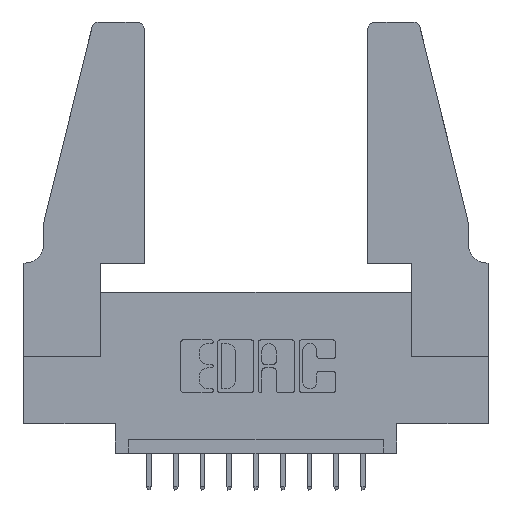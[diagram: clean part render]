
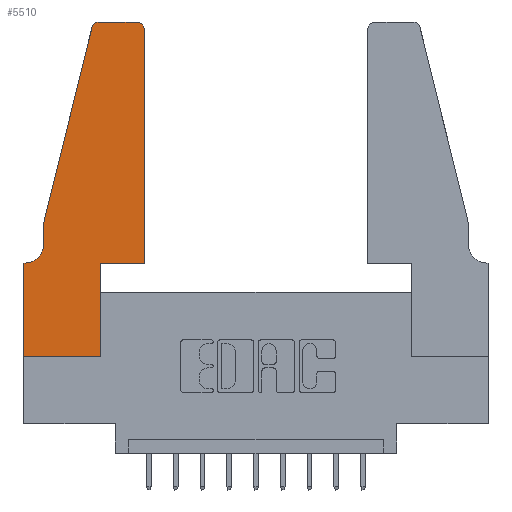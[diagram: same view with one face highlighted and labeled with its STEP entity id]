
A CAD part, top view. The second image highlights one B-rep face of the part: STEP entity #5510.
In plain terms, the highlighted planar face has unit normal (0, 0, 1).
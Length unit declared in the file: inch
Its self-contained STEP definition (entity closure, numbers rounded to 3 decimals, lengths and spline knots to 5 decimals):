
#42 = CARTESIAN_POINT ( 'NONE',  ( 0.4505, 1.22, 0.37 ) ) ;
#128 = VERTEX_POINT ( 'NONE', #8397 ) ;
#370 = EDGE_CURVE ( 'NONE', #12070, #12808, #12165, .T. ) ;
#937 = LINE ( 'NONE', #9481, #9171 ) ;
#1064 = CARTESIAN_POINT ( 'NONE',  ( 0.25487, 1.22718, 0.37 ) ) ;
#1077 = VERTEX_POINT ( 'NONE', #1064 ) ;
#1118 = EDGE_CURVE ( 'NONE', #5408, #12070, #3129, .T. ) ;
#1276 = EDGE_CURVE ( 'NONE', #12020, #12348, #7803, .T. ) ;
#1410 = VECTOR ( 'NONE', #4740, 39.37008 ) ;
#1493 = CARTESIAN_POINT ( 'NONE',  ( 0.0755, 0.42, 0.37 ) ) ;
#1813 = EDGE_CURVE ( 'NONE', #5186, #8409, #5020, .T. ) ;
#1976 = VECTOR ( 'NONE', #8343, 39.37008 ) ;
#2025 = CARTESIAN_POINT ( 'NONE',  ( 0., 0., 0.37 ) ) ;
#2161 = DIRECTION ( 'NONE',  ( 1., 0., 0. ) ) ;
#2251 = ORIENTED_EDGE ( 'NONE', *, *, #11714, .T. ) ;
#2435 = CARTESIAN_POINT ( 'NONE',  ( 0.284, 1.22, 0.37 ) ) ;
#3129 = LINE ( 'NONE', #2025, #11749 ) ;
#3147 = DIRECTION ( 'NONE',  ( -1., 0., 0. ) ) ;
#3372 = PLANE ( 'NONE',  #5221 ) ;
#3599 = DIRECTION ( 'NONE',  ( 1., 0., 0. ) ) ;
#4174 = CARTESIAN_POINT ( 'NONE',  ( 0.0055, 0.42, 0.37 ) ) ;
#4243 = DIRECTION ( 'NONE',  ( -1., 0., 0. ) ) ;
#4270 = FACE_OUTER_BOUND ( 'NONE', #7296, .T. ) ;
#4413 = EDGE_CURVE ( 'NONE', #128, #9980, #937, .T. ) ;
#4471 = DIRECTION ( 'NONE',  ( 1., 0., 0. ) ) ;
#4550 = DIRECTION ( 'NONE',  ( -1., 0., 0. ) ) ;
#4599 = CIRCLE ( 'NONE', #12306, 0.07 ) ;
#4655 = EDGE_CURVE ( 'NONE', #10819, #1077, #11586, .T. ) ;
#4688 = ORIENTED_EDGE ( 'NONE', *, *, #1276, .T. ) ;
#4740 = DIRECTION ( 'NONE',  ( 0., 1., 0. ) ) ;
#4826 = ORIENTED_EDGE ( 'NONE', *, *, #1813, .T. ) ;
#4910 = CARTESIAN_POINT ( 'NONE',  ( 0.4505, 0.35, 0.37 ) ) ;
#5020 = LINE ( 'NONE', #13416, #12423 ) ;
#5090 = LINE ( 'NONE', #13544, #12951 ) ;
#5111 = CARTESIAN_POINT ( 'NONE',  ( 0., 0., 0.37 ) ) ;
#5183 = EDGE_CURVE ( 'NONE', #13500, #12020, #6913, .T. ) ;
#5186 = VERTEX_POINT ( 'NONE', #13297 ) ;
#5187 = CARTESIAN_POINT ( 'NONE',  ( 0.0755, 0.5, 0.37 ) ) ;
#5221 = AXIS2_PLACEMENT_3D ( 'NONE', #5519, #13118, #4471 ) ;
#5408 = VERTEX_POINT ( 'NONE', #11573 ) ;
#5510 = ADVANCED_FACE ( 'NONE', ( #4270 ), #3372, .T. ) ;
#5519 = CARTESIAN_POINT ( 'NONE',  ( 0., 0.35, 0.37 ) ) ;
#5619 = AXIS2_PLACEMENT_3D ( 'NONE', #12609, #7411, #2161 ) ;
#5861 = ORIENTED_EDGE ( 'NONE', *, *, #5183, .T. ) ;
#6378 = DIRECTION ( 'NONE',  ( 0., -1., 0. ) ) ;
#6474 = DIRECTION ( 'NONE',  ( 1., 0., 0. ) ) ;
#6489 = ORIENTED_EDGE ( 'NONE', *, *, #11638, .T. ) ;
#6744 = AXIS2_PLACEMENT_3D ( 'NONE', #2435, #7743, #3599 ) ;
#6913 = LINE ( 'NONE', #4910, #10937 ) ;
#7193 = ORIENTED_EDGE ( 'NONE', *, *, #12477, .T. ) ;
#7207 = ORIENTED_EDGE ( 'NONE', *, *, #7664, .T. ) ;
#7296 = EDGE_LOOP ( 'NONE', ( #6489, #12398, #10601, #9295, #2251, #4826, #7207, #9597, #10043, #7193, #5861, #4688 ) ) ;
#7411 = DIRECTION ( 'NONE',  ( 0., 0., 1. ) ) ;
#7415 = CARTESIAN_POINT ( 'NONE',  ( 0.4505, 0.35, 0.37 ) ) ;
#7664 = EDGE_CURVE ( 'NONE', #8409, #5408, #10019, .T. ) ;
#7743 = DIRECTION ( 'NONE',  ( 0., 0., 1. ) ) ;
#7771 = EDGE_CURVE ( 'NONE', #1077, #128, #10290, .T. ) ;
#7803 = CIRCLE ( 'NONE', #5619, 0.03 ) ;
#7941 = VECTOR ( 'NONE', #6474, 39.37008 ) ;
#8343 = DIRECTION ( 'NONE',  ( -0.239, -0.971, 0. ) ) ;
#8382 = DIRECTION ( 'NONE',  ( 0., 0., -1. ) ) ;
#8397 = CARTESIAN_POINT ( 'NONE',  ( 0.0755, 0.5, 0.37 ) ) ;
#8409 = VERTEX_POINT ( 'NONE', #11754 ) ;
#9108 = DIRECTION ( 'NONE',  ( 0., 1., 0. ) ) ;
#9171 = VECTOR ( 'NONE', #6378, 39.37008 ) ;
#9243 = CARTESIAN_POINT ( 'NONE',  ( 0.4205, 1.25, 0.37 ) ) ;
#9295 = ORIENTED_EDGE ( 'NONE', *, *, #4413, .T. ) ;
#9481 = CARTESIAN_POINT ( 'NONE',  ( 0.0755, 0.5, 0.37 ) ) ;
#9512 = CARTESIAN_POINT ( 'NONE',  ( 0.4505, 0.35, 0.37 ) ) ;
#9597 = ORIENTED_EDGE ( 'NONE', *, *, #1118, .T. ) ;
#9980 = VERTEX_POINT ( 'NONE', #1493 ) ;
#10019 = LINE ( 'NONE', #5111, #13405 ) ;
#10043 = ORIENTED_EDGE ( 'NONE', *, *, #370, .T. ) ;
#10191 = CARTESIAN_POINT ( 'NONE',  ( 0.2865, 0.35, 0.37 ) ) ;
#10290 = LINE ( 'NONE', #5187, #1976 ) ;
#10440 = DIRECTION ( 'NONE',  ( 1., 0., 0. ) ) ;
#10493 = CARTESIAN_POINT ( 'NONE',  ( 0.284, 1.25, 0.37 ) ) ;
#10601 = ORIENTED_EDGE ( 'NONE', *, *, #7771, .T. ) ;
#10612 = LINE ( 'NONE', #9512, #7941 ) ;
#10819 = VERTEX_POINT ( 'NONE', #10493 ) ;
#10937 = VECTOR ( 'NONE', #9108, 39.37008 ) ;
#11337 = CARTESIAN_POINT ( 'NONE',  ( 0.2865, 0., 0.37 ) ) ;
#11573 = CARTESIAN_POINT ( 'NONE',  ( 0., 0., 0.37 ) ) ;
#11586 = CIRCLE ( 'NONE', #6744, 0.03 ) ;
#11638 = EDGE_CURVE ( 'NONE', #12348, #10819, #5090, .T. ) ;
#11714 = EDGE_CURVE ( 'NONE', #9980, #5186, #4599, .T. ) ;
#11749 = VECTOR ( 'NONE', #10440, 39.37008 ) ;
#11754 = CARTESIAN_POINT ( 'NONE',  ( 0., 0.35, 0.37 ) ) ;
#12020 = VERTEX_POINT ( 'NONE', #42 ) ;
#12070 = VERTEX_POINT ( 'NONE', #11337 ) ;
#12165 = LINE ( 'NONE', #10191, #1410 ) ;
#12306 = AXIS2_PLACEMENT_3D ( 'NONE', #4174, #8382, #3147 ) ;
#12307 = CARTESIAN_POINT ( 'NONE',  ( 0.2865, 0.35, 0.37 ) ) ;
#12348 = VERTEX_POINT ( 'NONE', #9243 ) ;
#12398 = ORIENTED_EDGE ( 'NONE', *, *, #4655, .T. ) ;
#12423 = VECTOR ( 'NONE', #4550, 39.37008 ) ;
#12477 = EDGE_CURVE ( 'NONE', #12808, #13500, #10612, .T. ) ;
#12609 = CARTESIAN_POINT ( 'NONE',  ( 0.4205, 1.22, 0.37 ) ) ;
#12808 = VERTEX_POINT ( 'NONE', #12307 ) ;
#12951 = VECTOR ( 'NONE', #4243, 39.37008 ) ;
#13118 = DIRECTION ( 'NONE',  ( 0., 0., 1. ) ) ;
#13297 = CARTESIAN_POINT ( 'NONE',  ( 0.0055, 0.35, 0.37 ) ) ;
#13405 = VECTOR ( 'NONE', #13503, 39.37008 ) ;
#13416 = CARTESIAN_POINT ( 'NONE',  ( 0.0755, 0.35, 0.37 ) ) ;
#13500 = VERTEX_POINT ( 'NONE', #7415 ) ;
#13503 = DIRECTION ( 'NONE',  ( 0., -1., 0. ) ) ;
#13544 = CARTESIAN_POINT ( 'NONE',  ( 0.2605, 1.25, 0.37 ) ) ;
